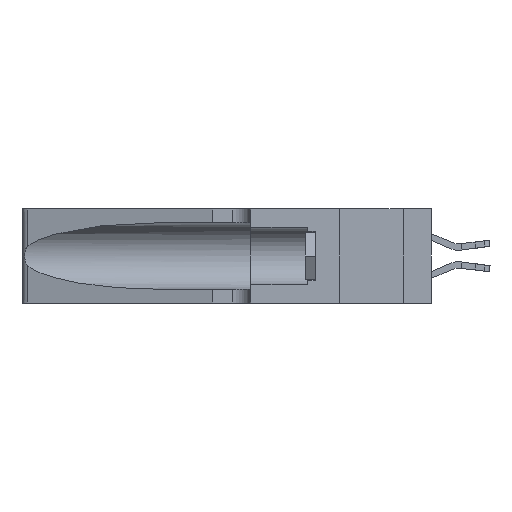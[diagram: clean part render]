
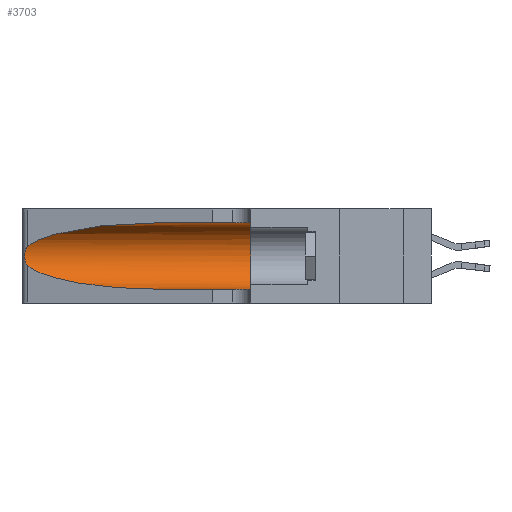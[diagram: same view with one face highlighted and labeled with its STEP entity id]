
A CAD part, left-side view. The second image highlights one B-rep face of the part: STEP entity #3703.
In plain terms, the highlighted cylindrical face has radius 3.308 mm (diameter 6.617 mm), a partial arc.
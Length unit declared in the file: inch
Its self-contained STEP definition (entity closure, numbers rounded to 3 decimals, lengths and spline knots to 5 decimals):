
#4 = VERTEX_POINT ( 'NONE', #20868 ) ;
#357 = ORIENTED_EDGE ( 'NONE', *, *, #3916, .T. ) ;
#790 = CARTESIAN_POINT ( 'NONE',  ( 0.26018, 1.23835, 0.19895 ) ) ;
#878 = CARTESIAN_POINT ( 'NONE',  ( 0.1305, 0.72297, 0.05475 ) ) ;
#1037 = CARTESIAN_POINT ( 'NONE',  ( 0.1305, 0.35, 0.185 ) ) ;
#1085 = CIRCLE ( 'NONE', #20394, 0.13025 ) ;
#1236 = VERTEX_POINT ( 'NONE', #10609 ) ;
#1367 = B_SPLINE_CURVE_WITH_KNOTS ( 'NONE', 3,
 ( #17297, #5973, #9303, #20452, #10964, #790, #12559, #2551, #14168, #4312, #15752, #6041, #17378, #7703 ),
 .UNSPECIFIED., .F., .F.,
 ( 4, 2, 2, 2, 2, 2, 4 ),
 ( 0., 0.00027, 0.00053, 0.00107, 0.0016, 0.00187, 0.00214 ),
 .UNSPECIFIED. ) ;
#1479 = EDGE_LOOP ( 'NONE', ( #19150, #10046, #357, #20970, #5562, #19993 ) ) ;
#1665 = DIRECTION ( 'NONE',  ( 0., -1., 0. ) ) ;
#2110 =( BOUNDED_CURVE ( )  B_SPLINE_CURVE ( 3, ( #4259, #9259, #6006, #17341 ),
 .UNSPECIFIED., .F., .F. ) 
 B_SPLINE_CURVE_WITH_KNOTS ( ( 4, 4 ),
 ( 1.5708, 2.84003 ),
 .UNSPECIFIED. ) 
 CURVE ( )  GEOMETRIC_REPRESENTATION_ITEM ( )  RATIONAL_B_SPLINE_CURVE ( ( 1., 0.87, 0.87, 1. ) ) 
 REPRESENTATION_ITEM ( '' )  );
#2551 = CARTESIAN_POINT ( 'NONE',  ( 0.26075, 1.23896, 0.178 ) ) ;
#2570 = CARTESIAN_POINT ( 'NONE',  ( 0.2373, 1.15595, 0.08982 ) ) ;
#2787 = DIRECTION ( 'NONE',  ( 0., 0., 1. ) ) ;
#2961 =( BOUNDED_CURVE ( )  B_SPLINE_CURVE ( 3, ( #11040, #2570, #17392, #878 ),
 .UNSPECIFIED., .F., .F. ) 
 B_SPLINE_CURVE_WITH_KNOTS ( ( 4, 4 ),
 ( 3.44316, 4.71239 ),
 .UNSPECIFIED. ) 
 CURVE ( )  GEOMETRIC_REPRESENTATION_ITEM ( )  RATIONAL_B_SPLINE_CURVE ( ( 1., 0.87, 0.87, 1. ) ) 
 REPRESENTATION_ITEM ( '' )  );
#3703 = ADVANCED_FACE ( 'NONE', ( #10628 ), #18615, .F. ) ;
#3916 = EDGE_CURVE ( 'NONE', #9702, #15638, #2961, .T. ) ;
#4259 = CARTESIAN_POINT ( 'NONE',  ( 0.1305, 0.72297, 0.31525 ) ) ;
#4312 = CARTESIAN_POINT ( 'NONE',  ( 0.25856, 1.23593, 0.16098 ) ) ;
#5461 = DIRECTION ( 'NONE',  ( 0., 0., -1. ) ) ;
#5562 = ORIENTED_EDGE ( 'NONE', *, *, #18436, .F. ) ;
#5568 = CARTESIAN_POINT ( 'NONE',  ( 0.1305, 0.35, 0.31525 ) ) ;
#5809 = VERTEX_POINT ( 'NONE', #5568 ) ;
#5973 = CARTESIAN_POINT ( 'NONE',  ( 0.25555, 1.22994, 0.2215 ) ) ;
#6006 = CARTESIAN_POINT ( 'NONE',  ( 0.2373, 1.15595, 0.28018 ) ) ;
#6041 = CARTESIAN_POINT ( 'NONE',  ( 0.25639, 1.23186, 0.15144 ) ) ;
#6268 = DIRECTION ( 'NONE',  ( 0., -1., 0. ) ) ;
#6797 = VERTEX_POINT ( 'NONE', #15922 ) ;
#6857 = CARTESIAN_POINT ( 'NONE',  ( 0.1305, 1.61858, 0.31525 ) ) ;
#7153 = DIRECTION ( 'NONE',  ( 0., -1., 0. ) ) ;
#7323 = AXIS2_PLACEMENT_3D ( 'NONE', #16847, #7153, #5461 ) ;
#7374 = EDGE_CURVE ( 'NONE', #15638, #6797, #11107, .T. ) ;
#7703 = CARTESIAN_POINT ( 'NONE',  ( 0.25487, 1.22718, 0.14631 ) ) ;
#7766 = LINE ( 'NONE', #6857, #11618 ) ;
#8894 = EDGE_CURVE ( 'NONE', #4, #1236, #2110, .T. ) ;
#9259 = CARTESIAN_POINT ( 'NONE',  ( 0.18966, 0.96281, 0.31525 ) ) ;
#9303 = CARTESIAN_POINT ( 'NONE',  ( 0.25639, 1.23184, 0.21858 ) ) ;
#9702 = VERTEX_POINT ( 'NONE', #14382 ) ;
#10046 = ORIENTED_EDGE ( 'NONE', *, *, #13261, .T. ) ;
#10609 = CARTESIAN_POINT ( 'NONE',  ( 0.25487, 1.22718, 0.22369 ) ) ;
#10628 = FACE_OUTER_BOUND ( 'NONE', #1479, .T. ) ;
#10964 = CARTESIAN_POINT ( 'NONE',  ( 0.25854, 1.2359, 0.20912 ) ) ;
#11040 = CARTESIAN_POINT ( 'NONE',  ( 0.25487, 1.22718, 0.14631 ) ) ;
#11107 = LINE ( 'NONE', #19164, #18581 ) ;
#11148 = EDGE_CURVE ( 'NONE', #4, #5809, #7766, .T. ) ;
#11618 = VECTOR ( 'NONE', #1665, 39.37008 ) ;
#12559 = CARTESIAN_POINT ( 'NONE',  ( 0.26075, 1.23896, 0.19203 ) ) ;
#12597 = CARTESIAN_POINT ( 'NONE',  ( 0.1305, 0.72297, 0.05475 ) ) ;
#12762 = DIRECTION ( 'NONE',  ( 0., 1., 0. ) ) ;
#13261 = EDGE_CURVE ( 'NONE', #1236, #9702, #1367, .T. ) ;
#14168 = CARTESIAN_POINT ( 'NONE',  ( 0.26017, 1.23833, 0.17102 ) ) ;
#14382 = CARTESIAN_POINT ( 'NONE',  ( 0.25487, 1.22718, 0.14631 ) ) ;
#15638 = VERTEX_POINT ( 'NONE', #12597 ) ;
#15752 = CARTESIAN_POINT ( 'NONE',  ( 0.25789, 1.23486, 0.15765 ) ) ;
#15922 = CARTESIAN_POINT ( 'NONE',  ( 0.1305, 0.35, 0.05475 ) ) ;
#16847 = CARTESIAN_POINT ( 'NONE',  ( 0.1305, 1.61858, 0.185 ) ) ;
#17297 = CARTESIAN_POINT ( 'NONE',  ( 0.25487, 1.22718, 0.22369 ) ) ;
#17341 = CARTESIAN_POINT ( 'NONE',  ( 0.25487, 1.22718, 0.22369 ) ) ;
#17378 = CARTESIAN_POINT ( 'NONE',  ( 0.25555, 1.22993, 0.14849 ) ) ;
#17392 = CARTESIAN_POINT ( 'NONE',  ( 0.18966, 0.96281, 0.05475 ) ) ;
#18436 = EDGE_CURVE ( 'NONE', #5809, #6797, #1085, .T. ) ;
#18581 = VECTOR ( 'NONE', #6268, 39.37008 ) ;
#18615 = CYLINDRICAL_SURFACE ( 'NONE', #7323, 0.13025 ) ;
#19150 = ORIENTED_EDGE ( 'NONE', *, *, #8894, .T. ) ;
#19164 = CARTESIAN_POINT ( 'NONE',  ( 0.1305, 1.61858, 0.05475 ) ) ;
#19993 = ORIENTED_EDGE ( 'NONE', *, *, #11148, .F. ) ;
#20394 = AXIS2_PLACEMENT_3D ( 'NONE', #1037, #12762, #2787 ) ;
#20452 = CARTESIAN_POINT ( 'NONE',  ( 0.25787, 1.23484, 0.2124 ) ) ;
#20868 = CARTESIAN_POINT ( 'NONE',  ( 0.1305, 0.72297, 0.31525 ) ) ;
#20970 = ORIENTED_EDGE ( 'NONE', *, *, #7374, .T. ) ;
